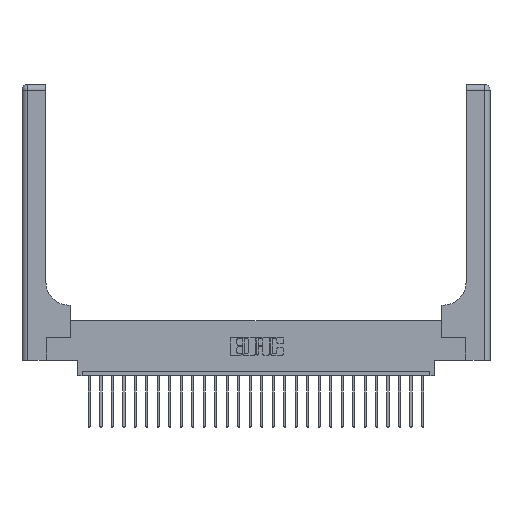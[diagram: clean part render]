
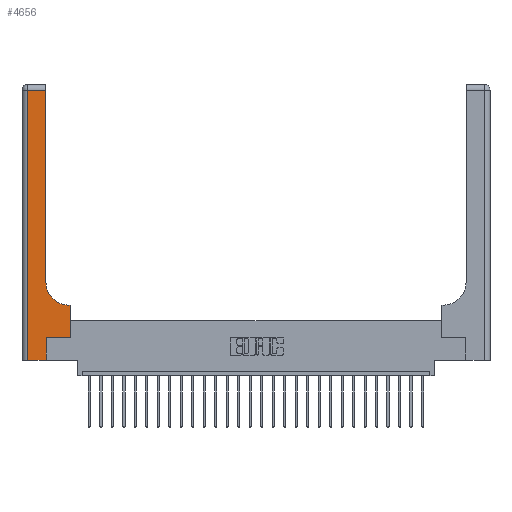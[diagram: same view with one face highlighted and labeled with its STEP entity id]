
A CAD part, top view. The second image highlights one B-rep face of the part: STEP entity #4656.
In plain terms, the highlighted planar face has unit normal (0, 0, 1).
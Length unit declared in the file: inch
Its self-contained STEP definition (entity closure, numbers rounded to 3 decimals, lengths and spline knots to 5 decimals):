
#104 = LINE ( 'NONE', #16124, #15849 ) ;
#407 = CARTESIAN_POINT ( 'NONE',  ( 0.528, 0.25, 0.37 ) ) ;
#515 = DIRECTION ( 'NONE',  ( -1., 0., 0. ) ) ;
#541 = LINE ( 'NONE', #407, #11916 ) ;
#639 = PLANE ( 'NONE',  #20232 ) ;
#1336 = DIRECTION ( 'NONE',  ( 1., 0., 0. ) ) ;
#1428 = DIRECTION ( 'NONE',  ( 0., -1., 0. ) ) ;
#1493 = CARTESIAN_POINT ( 'NONE',  ( 0.528, 0.6, 0.37 ) ) ;
#1601 = LINE ( 'NONE', #25415, #18317 ) ;
#2104 = EDGE_CURVE ( 'NONE', #11715, #7424, #104, .T. ) ;
#2454 = EDGE_CURVE ( 'NONE', #12128, #24213, #16065, .T. ) ;
#2779 = EDGE_CURVE ( 'NONE', #7424, #4797, #4686, .T. ) ;
#2916 = ORIENTED_EDGE ( 'NONE', *, *, #3222, .T. ) ;
#3222 = EDGE_CURVE ( 'NONE', #4797, #20743, #13637, .T. ) ;
#4656 = ADVANCED_FACE ( 'NONE', ( #6278 ), #639, .F. ) ;
#4686 = CIRCLE ( 'NONE', #18968, 0.25 ) ;
#4797 = VERTEX_POINT ( 'NONE', #11134 ) ;
#5172 = ORIENTED_EDGE ( 'NONE', *, *, #15736, .T. ) ;
#6278 = FACE_OUTER_BOUND ( 'NONE', #16661, .T. ) ;
#7103 = DIRECTION ( 'NONE',  ( 0., 0., -1. ) ) ;
#7424 = VERTEX_POINT ( 'NONE', #10560 ) ;
#7545 = VERTEX_POINT ( 'NONE', #19589 ) ;
#8705 = ORIENTED_EDGE ( 'NONE', *, *, #2104, .T. ) ;
#8905 = DIRECTION ( 'NONE',  ( 1., 0., 0. ) ) ;
#9434 = DIRECTION ( 'NONE',  ( 0., 1., 0. ) ) ;
#10529 = ORIENTED_EDGE ( 'NONE', *, *, #20569, .T. ) ;
#10560 = CARTESIAN_POINT ( 'NONE',  ( 0.51, 0.6, 0.37 ) ) ;
#11134 = CARTESIAN_POINT ( 'NONE',  ( 0.26, 0.85, 0.37 ) ) ;
#11423 = CARTESIAN_POINT ( 'NONE',  ( 0.26, 3., 0.37 ) ) ;
#11715 = VERTEX_POINT ( 'NONE', #1493 ) ;
#11916 = VECTOR ( 'NONE', #16443, 39.37008 ) ;
#12115 = CARTESIAN_POINT ( 'NONE',  ( 0., 0., 0.37 ) ) ;
#12128 = VERTEX_POINT ( 'NONE', #25144 ) ;
#12578 = CARTESIAN_POINT ( 'NONE',  ( 0.265, 0.25, 0.37 ) ) ;
#12719 = CARTESIAN_POINT ( 'NONE',  ( 0.06, 2.94, 0.37 ) ) ;
#13098 = CARTESIAN_POINT ( 'NONE',  ( 0.265, 0.25, 0.37 ) ) ;
#13381 = CARTESIAN_POINT ( 'NONE',  ( 0.06, 3., 0.37 ) ) ;
#13580 = CARTESIAN_POINT ( 'NONE',  ( 0., 2.94, 0.37 ) ) ;
#13637 = LINE ( 'NONE', #11423, #19398 ) ;
#13660 = VECTOR ( 'NONE', #21369, 39.37008 ) ;
#14308 = CARTESIAN_POINT ( 'NONE',  ( 0., 3., 0.37 ) ) ;
#14799 = EDGE_CURVE ( 'NONE', #21118, #7545, #20756, .T. ) ;
#15336 = EDGE_CURVE ( 'NONE', #20743, #21976, #21236, .T. ) ;
#15736 = EDGE_CURVE ( 'NONE', #24213, #21118, #1601, .T. ) ;
#15849 = VECTOR ( 'NONE', #22204, 39.37008 ) ;
#16065 = LINE ( 'NONE', #12115, #16687 ) ;
#16124 = CARTESIAN_POINT ( 'NONE',  ( 0.26, 0.6, 0.37 ) ) ;
#16443 = DIRECTION ( 'NONE',  ( 0., 1., 0. ) ) ;
#16661 = EDGE_LOOP ( 'NONE', ( #2916, #16808, #18296, #24776, #5172, #17598, #10529, #8705, #25828 ) ) ;
#16687 = VECTOR ( 'NONE', #21991, 39.37008 ) ;
#16808 = ORIENTED_EDGE ( 'NONE', *, *, #15336, .T. ) ;
#17361 = CARTESIAN_POINT ( 'NONE',  ( 0.51, 0.85, 0.37 ) ) ;
#17598 = ORIENTED_EDGE ( 'NONE', *, *, #14799, .T. ) ;
#18296 = ORIENTED_EDGE ( 'NONE', *, *, #22145, .T. ) ;
#18317 = VECTOR ( 'NONE', #19363, 39.37008 ) ;
#18968 = AXIS2_PLACEMENT_3D ( 'NONE', #17361, #7103, #1336 ) ;
#19004 = CARTESIAN_POINT ( 'NONE',  ( 0.265, 0., 0.37 ) ) ;
#19363 = DIRECTION ( 'NONE',  ( 0., 1., 0. ) ) ;
#19398 = VECTOR ( 'NONE', #9434, 39.37008 ) ;
#19535 = VECTOR ( 'NONE', #8905, 39.37008 ) ;
#19569 = LINE ( 'NONE', #13381, #20445 ) ;
#19589 = CARTESIAN_POINT ( 'NONE',  ( 0.528, 0.25, 0.37 ) ) ;
#20232 = AXIS2_PLACEMENT_3D ( 'NONE', #14308, #22350, #515 ) ;
#20445 = VECTOR ( 'NONE', #1428, 39.37008 ) ;
#20569 = EDGE_CURVE ( 'NONE', #7545, #11715, #541, .T. ) ;
#20743 = VERTEX_POINT ( 'NONE', #23410 ) ;
#20756 = LINE ( 'NONE', #12578, #19535 ) ;
#21118 = VERTEX_POINT ( 'NONE', #13098 ) ;
#21236 = LINE ( 'NONE', #13580, #13660 ) ;
#21369 = DIRECTION ( 'NONE',  ( -1., 0., 0. ) ) ;
#21976 = VERTEX_POINT ( 'NONE', #12719 ) ;
#21991 = DIRECTION ( 'NONE',  ( 1., 0., 0. ) ) ;
#22145 = EDGE_CURVE ( 'NONE', #21976, #12128, #19569, .T. ) ;
#22204 = DIRECTION ( 'NONE',  ( -1., 0., 0. ) ) ;
#22350 = DIRECTION ( 'NONE',  ( 0., 0., -1. ) ) ;
#23410 = CARTESIAN_POINT ( 'NONE',  ( 0.26, 2.94, 0.37 ) ) ;
#24213 = VERTEX_POINT ( 'NONE', #19004 ) ;
#24776 = ORIENTED_EDGE ( 'NONE', *, *, #2454, .T. ) ;
#25144 = CARTESIAN_POINT ( 'NONE',  ( 0.06, 0., 0.37 ) ) ;
#25415 = CARTESIAN_POINT ( 'NONE',  ( 0.265, 0., 0.37 ) ) ;
#25828 = ORIENTED_EDGE ( 'NONE', *, *, #2779, .T. ) ;
